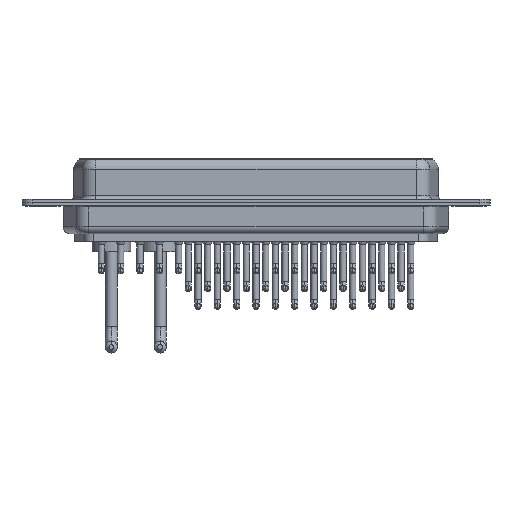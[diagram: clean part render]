
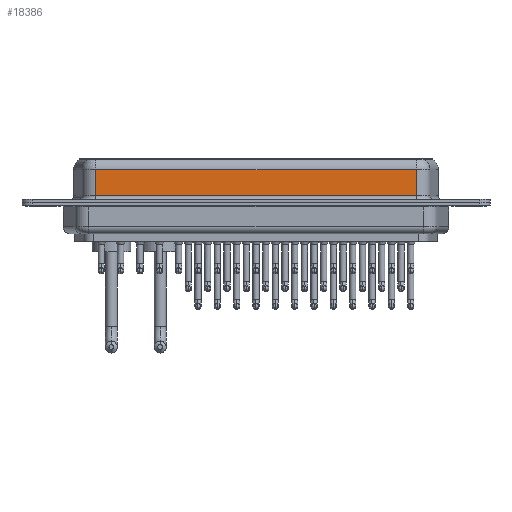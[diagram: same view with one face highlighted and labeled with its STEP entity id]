
A CAD part, front view. The second image highlights one B-rep face of the part: STEP entity #18386.
In plain terms, the highlighted planar face has unit normal (0, -1, 0).
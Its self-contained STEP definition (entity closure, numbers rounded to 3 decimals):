
#1520 = VECTOR ( 'NONE', #28510, 1000. ) ;
#1787 = DIRECTION ( 'NONE',  ( -1., 0., 0. ) ) ;
#2216 = CARTESIAN_POINT ( 'NONE',  ( 7.59, -5.375, 6.4 ) ) ;
#2491 = DIRECTION ( 'NONE',  ( 0., 0., -1. ) ) ;
#2918 = EDGE_CURVE ( 'NONE', #7795, #29523, #28010, .T. ) ;
#3032 = CARTESIAN_POINT ( 'NONE',  ( 7.59, -5.375, 0.9 ) ) ;
#4795 = CARTESIAN_POINT ( 'NONE',  ( 53.41, -5.375, 0.9 ) ) ;
#5673 = FACE_OUTER_BOUND ( 'NONE', #29569, .T. ) ;
#7052 = LINE ( 'NONE', #2216, #1520 ) ;
#7795 = VERTEX_POINT ( 'NONE', #17257 ) ;
#9247 = CARTESIAN_POINT ( 'NONE',  ( 53.41, -5.375, 0.9 ) ) ;
#11813 = CARTESIAN_POINT ( 'NONE',  ( 53.41, -5.375, 6.4 ) ) ;
#11873 = ORIENTED_EDGE ( 'NONE', *, *, #21316, .T. ) ;
#13793 = ORIENTED_EDGE ( 'NONE', *, *, #13849, .T. ) ;
#13849 = EDGE_CURVE ( 'NONE', #7795, #28565, #20619, .T. ) ;
#17037 = ORIENTED_EDGE ( 'NONE', *, *, #18981, .T. ) ;
#17257 = CARTESIAN_POINT ( 'NONE',  ( 53.41, -5.375, 4.65 ) ) ;
#17628 = ORIENTED_EDGE ( 'NONE', *, *, #2918, .F. ) ;
#18373 = DIRECTION ( 'NONE',  ( 0., 0., 1. ) ) ;
#18386 = ADVANCED_FACE ( 'NONE', ( #5673 ), #20703, .F. ) ;
#18794 = LINE ( 'NONE', #4795, #29686 ) ;
#18981 = EDGE_CURVE ( 'NONE', #29828, #29523, #18794, .T. ) ;
#19831 = DIRECTION ( 'NONE',  ( 0., 1., 0. ) ) ;
#20619 = LINE ( 'NONE', #22632, #26018 ) ;
#20703 = PLANE ( 'NONE',  #22318 ) ;
#21316 = EDGE_CURVE ( 'NONE', #28565, #29828, #7052, .T. ) ;
#22318 = AXIS2_PLACEMENT_3D ( 'NONE', #27998, #19831, #18373 ) ;
#22632 = CARTESIAN_POINT ( 'NONE',  ( 53.41, -5.375, 4.65 ) ) ;
#22777 = VECTOR ( 'NONE', #2491, 1000. ) ;
#25405 = CARTESIAN_POINT ( 'NONE',  ( 7.59, -5.375, 4.65 ) ) ;
#26018 = VECTOR ( 'NONE', #1787, 1000. ) ;
#27998 = CARTESIAN_POINT ( 'NONE',  ( 53.41, -5.375, 6.4 ) ) ;
#28010 = LINE ( 'NONE', #11813, #22777 ) ;
#28510 = DIRECTION ( 'NONE',  ( 0., 0., -1. ) ) ;
#28565 = VERTEX_POINT ( 'NONE', #25405 ) ;
#29523 = VERTEX_POINT ( 'NONE', #9247 ) ;
#29569 = EDGE_LOOP ( 'NONE', ( #17628, #13793, #11873, #17037 ) ) ;
#29686 = VECTOR ( 'NONE', #30588, 1000. ) ;
#29828 = VERTEX_POINT ( 'NONE', #3032 ) ;
#30588 = DIRECTION ( 'NONE',  ( 1., 0., 0. ) ) ;
